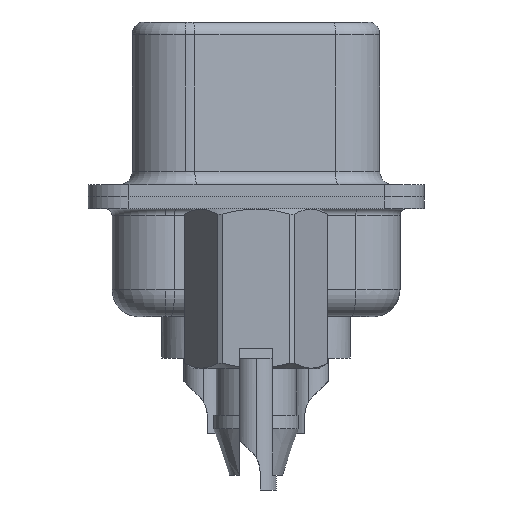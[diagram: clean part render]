
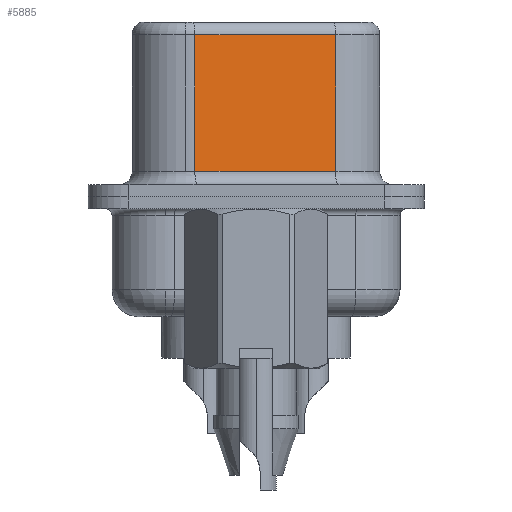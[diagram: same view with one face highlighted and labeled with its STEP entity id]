
A CAD part, left-side view. The second image highlights one B-rep face of the part: STEP entity #5885.
In plain terms, the highlighted planar face has unit normal (-0.985, -0.174, 0).
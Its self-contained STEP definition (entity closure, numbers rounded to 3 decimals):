
#53 = ORIENTED_EDGE ( 'NONE', *, *, #19846, .T. ) ;
#211 = VECTOR ( 'NONE', #15245, 1000. ) ;
#763 = LINE ( 'NONE', #7077, #12647 ) ;
#1298 = CARTESIAN_POINT ( 'NONE',  ( 4.546, -2.987, 6.57 ) ) ;
#1783 = EDGE_CURVE ( 'NONE', #20227, #13316, #6640, .T. ) ;
#4542 = DIRECTION ( 'NONE',  ( -0.174, 0.985, 0. ) ) ;
#5408 = CARTESIAN_POINT ( 'NONE',  ( 4.546, -2.987, 6.07 ) ) ;
#5885 = ADVANCED_FACE ( 'NONE', ( #11556 ), #18919, .F. ) ;
#6528 = CARTESIAN_POINT ( 'NONE',  ( 4.546, -2.987, 6.07 ) ) ;
#6640 = LINE ( 'NONE', #19408, #18414 ) ;
#6869 = DIRECTION ( 'NONE',  ( 0., 0., -1. ) ) ;
#7077 = CARTESIAN_POINT ( 'NONE',  ( 3.615, 2.293, 6.57 ) ) ;
#7567 = CARTESIAN_POINT ( 'NONE',  ( 4.546, -2.987, 6.57 ) ) ;
#7684 = ORIENTED_EDGE ( 'NONE', *, *, #16644, .F. ) ;
#7812 = DIRECTION ( 'NONE',  ( 0.985, 0.174, 0. ) ) ;
#9164 = CARTESIAN_POINT ( 'NONE',  ( 4.546, -2.987, 0.95 ) ) ;
#9736 = EDGE_LOOP ( 'NONE', ( #7684, #19476, #53, #20067 ) ) ;
#9872 = VERTEX_POINT ( 'NONE', #13640 ) ;
#11556 = FACE_OUTER_BOUND ( 'NONE', #9736, .T. ) ;
#11726 = DIRECTION ( 'NONE',  ( 0.174, -0.985, 0. ) ) ;
#11965 = CARTESIAN_POINT ( 'NONE',  ( 3.615, 2.293, 0.95 ) ) ;
#12647 = VECTOR ( 'NONE', #6869, 1000. ) ;
#12797 = LINE ( 'NONE', #7567, #14234 ) ;
#13272 = LINE ( 'NONE', #5408, #211 ) ;
#13316 = VERTEX_POINT ( 'NONE', #9164 ) ;
#13640 = CARTESIAN_POINT ( 'NONE',  ( 3.615, 2.293, 6.07 ) ) ;
#14234 = VECTOR ( 'NONE', #15727, 1000. ) ;
#15245 = DIRECTION ( 'NONE',  ( -0.174, 0.985, 0. ) ) ;
#15727 = DIRECTION ( 'NONE',  ( 0., 0., -1. ) ) ;
#16644 = EDGE_CURVE ( 'NONE', #16745, #13316, #12797, .T. ) ;
#16745 = VERTEX_POINT ( 'NONE', #6528 ) ;
#17286 = AXIS2_PLACEMENT_3D ( 'NONE', #1298, #7812, #4542 ) ;
#17847 = EDGE_CURVE ( 'NONE', #16745, #9872, #13272, .T. ) ;
#18414 = VECTOR ( 'NONE', #11726, 1000. ) ;
#18919 = PLANE ( 'NONE',  #17286 ) ;
#19408 = CARTESIAN_POINT ( 'NONE',  ( 4.546, -2.987, 0.95 ) ) ;
#19476 = ORIENTED_EDGE ( 'NONE', *, *, #17847, .T. ) ;
#19846 = EDGE_CURVE ( 'NONE', #9872, #20227, #763, .T. ) ;
#20067 = ORIENTED_EDGE ( 'NONE', *, *, #1783, .T. ) ;
#20227 = VERTEX_POINT ( 'NONE', #11965 ) ;
